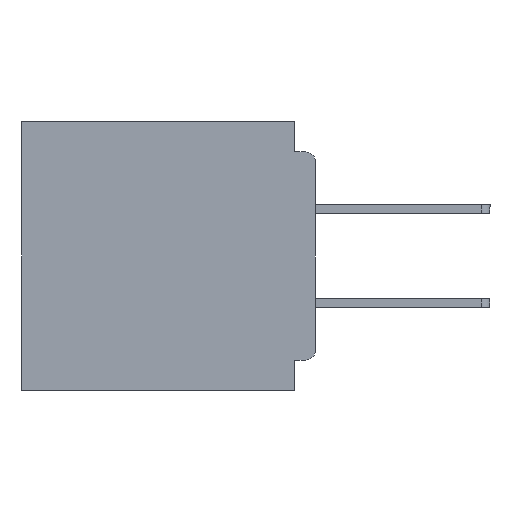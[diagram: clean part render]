
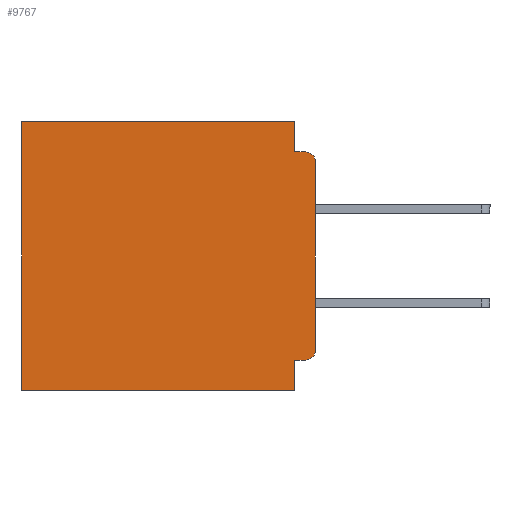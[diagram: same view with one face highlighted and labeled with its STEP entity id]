
A CAD part, left-side view. The second image highlights one B-rep face of the part: STEP entity #9767.
In plain terms, the highlighted planar face has unit normal (-1, 0, 0).
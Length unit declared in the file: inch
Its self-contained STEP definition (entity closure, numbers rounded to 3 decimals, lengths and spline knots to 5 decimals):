
#80 = VERTEX_POINT ( 'NONE', #1764 ) ;
#742 = LINE ( 'NONE', #27168, #7878 ) ;
#1254 = CARTESIAN_POINT ( 'NONE',  ( 0.3, 0., -0.34 ) ) ;
#1572 = ORIENTED_EDGE ( 'NONE', *, *, #16559, .T. ) ;
#1611 = EDGE_CURVE ( 'NONE', #35282, #18581, #13000, .T. ) ;
#1764 = CARTESIAN_POINT ( 'NONE',  ( 0.3, 0.031, -0.045 ) ) ;
#2892 = EDGE_CURVE ( 'NONE', #80, #38228, #30731, .T. ) ;
#3326 = DIRECTION ( 'NONE',  ( -1., 0., 0. ) ) ;
#4107 = LINE ( 'NONE', #30864, #19147 ) ;
#5195 = DIRECTION ( 'NONE',  ( 0., 0., -1. ) ) ;
#5638 = ORIENTED_EDGE ( 'NONE', *, *, #26729, .F. ) ;
#7878 = VECTOR ( 'NONE', #12305, 39.37008 ) ;
#7906 = CARTESIAN_POINT ( 'NONE',  ( 0.3, 0.015, -0.355 ) ) ;
#7969 = CARTESIAN_POINT ( 'NONE',  ( 0.3, 0.031, 0. ) ) ;
#8070 = ORIENTED_EDGE ( 'NONE', *, *, #21909, .F. ) ;
#9705 = CARTESIAN_POINT ( 'NONE',  ( 0.3, 0.015, -0.045 ) ) ;
#9767 = ADVANCED_FACE ( 'NONE', ( #37863 ), #30152, .F. ) ;
#12295 = VECTOR ( 'NONE', #37991, 39.37008 ) ;
#12305 = DIRECTION ( 'NONE',  ( 0., 1., 0. ) ) ;
#12604 = EDGE_CURVE ( 'NONE', #18642, #21601, #15350, .T. ) ;
#12791 = CARTESIAN_POINT ( 'NONE',  ( 0.3, 0., -0.4 ) ) ;
#13000 = CIRCLE ( 'NONE', #29198, 0.015 ) ;
#13496 = DIRECTION ( 'NONE',  ( 0., 0., -1. ) ) ;
#13716 = EDGE_CURVE ( 'NONE', #32200, #38228, #27054, .T. ) ;
#14230 = ORIENTED_EDGE ( 'NONE', *, *, #2892, .F. ) ;
#14313 = ORIENTED_EDGE ( 'NONE', *, *, #17765, .F. ) ;
#15350 = LINE ( 'NONE', #12791, #25243 ) ;
#16038 = CARTESIAN_POINT ( 'NONE',  ( 0.3, 0., 0. ) ) ;
#16559 = EDGE_CURVE ( 'NONE', #28831, #37717, #20177, .T. ) ;
#16560 = VECTOR ( 'NONE', #13496, 39.37008 ) ;
#17158 = AXIS2_PLACEMENT_3D ( 'NONE', #21354, #3326, #24420 ) ;
#17329 = CARTESIAN_POINT ( 'NONE',  ( 0.3, 0., -0.06 ) ) ;
#17523 = ORIENTED_EDGE ( 'NONE', *, *, #1611, .T. ) ;
#17765 = EDGE_CURVE ( 'NONE', #35282, #36111, #742, .T. ) ;
#18060 = DIRECTION ( 'NONE',  ( 0., -1., 0. ) ) ;
#18294 = VECTOR ( 'NONE', #36944, 39.37008 ) ;
#18581 = VERTEX_POINT ( 'NONE', #1254 ) ;
#18642 = VERTEX_POINT ( 'NONE', #31587 ) ;
#19147 = VECTOR ( 'NONE', #33788, 39.37008 ) ;
#20177 = LINE ( 'NONE', #16038, #18294 ) ;
#20278 = EDGE_LOOP ( 'NONE', ( #32522, #35586, #14230, #5638, #1572, #27432, #31742, #8070, #14313, #17523 ) ) ;
#21022 = EDGE_CURVE ( 'NONE', #37717, #21601, #35064, .T. ) ;
#21354 = CARTESIAN_POINT ( 'NONE',  ( 0.3, 0.015, -0.06 ) ) ;
#21601 = VERTEX_POINT ( 'NONE', #29500 ) ;
#21832 = VECTOR ( 'NONE', #18060, 39.37008 ) ;
#21909 = EDGE_CURVE ( 'NONE', #36111, #18642, #4107, .T. ) ;
#22453 = CARTESIAN_POINT ( 'NONE',  ( 0.3, 0.031, 0. ) ) ;
#23236 = CARTESIAN_POINT ( 'NONE',  ( 0.3, 0.437, -0.4 ) ) ;
#24420 = DIRECTION ( 'NONE',  ( 0., 0., -1. ) ) ;
#24583 = LINE ( 'NONE', #22453, #16560 ) ;
#25243 = VECTOR ( 'NONE', #30869, 39.37008 ) ;
#25453 = CARTESIAN_POINT ( 'NONE',  ( 0.3, 0., -0.045 ) ) ;
#26729 = EDGE_CURVE ( 'NONE', #28831, #80, #24583, .T. ) ;
#27054 = CIRCLE ( 'NONE', #17158, 0.015 ) ;
#27168 = CARTESIAN_POINT ( 'NONE',  ( 0.3, 0., -0.355 ) ) ;
#27432 = ORIENTED_EDGE ( 'NONE', *, *, #21022, .T. ) ;
#28206 = VECTOR ( 'NONE', #5195, 39.37008 ) ;
#28831 = VERTEX_POINT ( 'NONE', #7969 ) ;
#29198 = AXIS2_PLACEMENT_3D ( 'NONE', #32657, #32341, #32333 ) ;
#29224 = CARTESIAN_POINT ( 'NONE',  ( 0.3, 0., -0.4 ) ) ;
#29500 = CARTESIAN_POINT ( 'NONE',  ( 0.3, 0.437, -0.4 ) ) ;
#30099 = DIRECTION ( 'NONE',  ( 0., 0., -1. ) ) ;
#30146 = DIRECTION ( 'NONE',  ( 1., 0., 0. ) ) ;
#30152 = PLANE ( 'NONE',  #33557 ) ;
#30276 = CARTESIAN_POINT ( 'NONE',  ( 0.3, 0., -0.4 ) ) ;
#30731 = LINE ( 'NONE', #25453, #21832 ) ;
#30864 = CARTESIAN_POINT ( 'NONE',  ( 0.3, 0.031, -0.4 ) ) ;
#30869 = DIRECTION ( 'NONE',  ( 0., 1., 0. ) ) ;
#31587 = CARTESIAN_POINT ( 'NONE',  ( 0.3, 0.031, -0.4 ) ) ;
#31742 = ORIENTED_EDGE ( 'NONE', *, *, #12604, .F. ) ;
#32200 = VERTEX_POINT ( 'NONE', #17329 ) ;
#32333 = DIRECTION ( 'NONE',  ( 0., 0., -1. ) ) ;
#32341 = DIRECTION ( 'NONE',  ( -1., 0., 0. ) ) ;
#32522 = ORIENTED_EDGE ( 'NONE', *, *, #33310, .F. ) ;
#32581 = CARTESIAN_POINT ( 'NONE',  ( 0.3, 0.031, -0.355 ) ) ;
#32657 = CARTESIAN_POINT ( 'NONE',  ( 0.3, 0.015, -0.34 ) ) ;
#33310 = EDGE_CURVE ( 'NONE', #32200, #18581, #36035, .T. ) ;
#33557 = AXIS2_PLACEMENT_3D ( 'NONE', #30276, #30146, #30099 ) ;
#33788 = DIRECTION ( 'NONE',  ( 0., 0., -1. ) ) ;
#34128 = CARTESIAN_POINT ( 'NONE',  ( 0.3, 0.437, 0. ) ) ;
#35064 = LINE ( 'NONE', #23236, #28206 ) ;
#35282 = VERTEX_POINT ( 'NONE', #7906 ) ;
#35586 = ORIENTED_EDGE ( 'NONE', *, *, #13716, .T. ) ;
#36035 = LINE ( 'NONE', #29224, #12295 ) ;
#36111 = VERTEX_POINT ( 'NONE', #32581 ) ;
#36944 = DIRECTION ( 'NONE',  ( 0., 1., 0. ) ) ;
#37717 = VERTEX_POINT ( 'NONE', #34128 ) ;
#37863 = FACE_OUTER_BOUND ( 'NONE', #20278, .T. ) ;
#37991 = DIRECTION ( 'NONE',  ( 0., 0., -1. ) ) ;
#38228 = VERTEX_POINT ( 'NONE', #9705 ) ;
